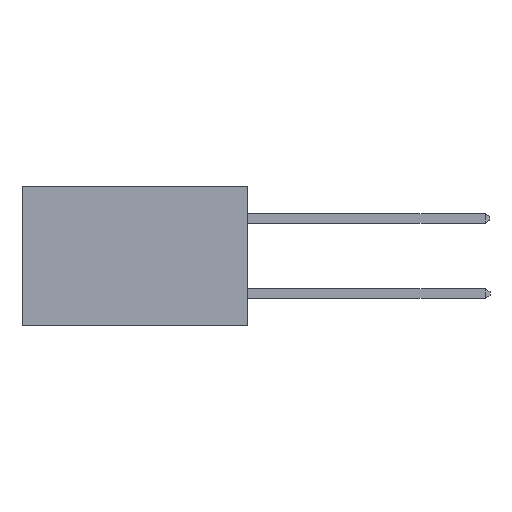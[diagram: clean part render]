
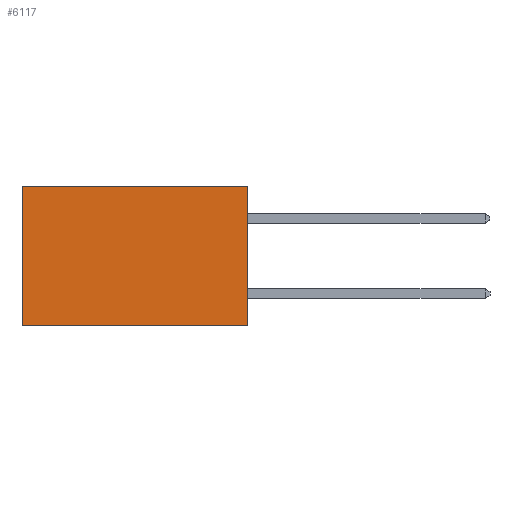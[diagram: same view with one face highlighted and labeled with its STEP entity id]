
A CAD part, left-side view. The second image highlights one B-rep face of the part: STEP entity #6117.
In plain terms, the highlighted planar face has unit normal (-1, 0, 0).
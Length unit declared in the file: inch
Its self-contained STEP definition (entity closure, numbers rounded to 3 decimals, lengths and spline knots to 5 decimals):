
#2 = LINE ( 'NONE', #1778, #3790 ) ;
#51 = VERTEX_POINT ( 'NONE', #5327 ) ;
#599 = DIRECTION ( 'NONE',  ( 0., 0., -1. ) ) ;
#784 = EDGE_CURVE ( 'NONE', #7921, #3235, #7162, .T. ) ;
#1654 = VECTOR ( 'NONE', #7307, 39.37008 ) ;
#1778 = CARTESIAN_POINT ( 'NONE',  ( 0.2615, 0., -0.37 ) ) ;
#1890 = ORIENTED_EDGE ( 'NONE', *, *, #7832, .F. ) ;
#2615 = VECTOR ( 'NONE', #4635, 39.37008 ) ;
#2833 = EDGE_LOOP ( 'NONE', ( #3396, #8750, #1890, #9490 ) ) ;
#2927 = CARTESIAN_POINT ( 'NONE',  ( 0.2615, 0.6, 0. ) ) ;
#2954 = CARTESIAN_POINT ( 'NONE',  ( 0.2615, 0., -0.37 ) ) ;
#3235 = VERTEX_POINT ( 'NONE', #6409 ) ;
#3396 = ORIENTED_EDGE ( 'NONE', *, *, #7646, .T. ) ;
#3753 = CARTESIAN_POINT ( 'NONE',  ( 0.2615, 0., -0.37 ) ) ;
#3790 = VECTOR ( 'NONE', #7834, 39.37008 ) ;
#3892 = EDGE_CURVE ( 'NONE', #51, #6210, #8467, .T. ) ;
#4371 = CARTESIAN_POINT ( 'NONE',  ( 0.2615, 0., -0.37 ) ) ;
#4635 = DIRECTION ( 'NONE',  ( 0., 1., 0. ) ) ;
#4658 = FACE_OUTER_BOUND ( 'NONE', #2833, .T. ) ;
#5140 = DIRECTION ( 'NONE',  ( 1., 0., 0. ) ) ;
#5327 = CARTESIAN_POINT ( 'NONE',  ( 0.2615, 0., 0. ) ) ;
#5589 = AXIS2_PLACEMENT_3D ( 'NONE', #4371, #5140, #599 ) ;
#5610 = LINE ( 'NONE', #7340, #1654 ) ;
#5671 = VECTOR ( 'NONE', #8646, 39.37008 ) ;
#6117 = ADVANCED_FACE ( 'NONE', ( #4658 ), #8914, .F. ) ;
#6210 = VERTEX_POINT ( 'NONE', #2927 ) ;
#6338 = CARTESIAN_POINT ( 'NONE',  ( 0.2615, 0., 0. ) ) ;
#6409 = CARTESIAN_POINT ( 'NONE',  ( 0.2615, 0.6, -0.37 ) ) ;
#7162 = LINE ( 'NONE', #3753, #2615 ) ;
#7307 = DIRECTION ( 'NONE',  ( 0., 0., -1. ) ) ;
#7340 = CARTESIAN_POINT ( 'NONE',  ( 0.2615, 0.6, -0.37 ) ) ;
#7646 = EDGE_CURVE ( 'NONE', #6210, #3235, #5610, .T. ) ;
#7832 = EDGE_CURVE ( 'NONE', #51, #7921, #2, .T. ) ;
#7834 = DIRECTION ( 'NONE',  ( 0., 0., -1. ) ) ;
#7921 = VERTEX_POINT ( 'NONE', #2954 ) ;
#8467 = LINE ( 'NONE', #6338, #5671 ) ;
#8646 = DIRECTION ( 'NONE',  ( 0., 1., 0. ) ) ;
#8750 = ORIENTED_EDGE ( 'NONE', *, *, #784, .F. ) ;
#8914 = PLANE ( 'NONE',  #5589 ) ;
#9490 = ORIENTED_EDGE ( 'NONE', *, *, #3892, .T. ) ;
